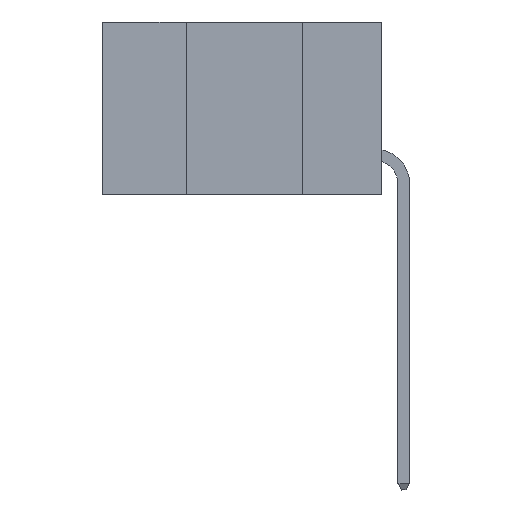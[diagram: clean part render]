
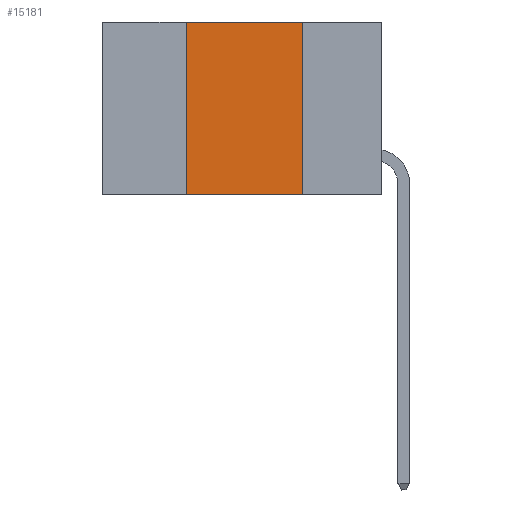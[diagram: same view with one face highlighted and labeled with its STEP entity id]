
A CAD part, left-side view. The second image highlights one B-rep face of the part: STEP entity #15181.
In plain terms, the highlighted planar face has unit normal (-1, 0, 0).
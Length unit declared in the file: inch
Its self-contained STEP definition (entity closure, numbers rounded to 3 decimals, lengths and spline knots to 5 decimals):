
#369 = VECTOR ( 'NONE', #15981, 39.37008 ) ;
#800 = DIRECTION ( 'NONE',  ( 0., 0., -1. ) ) ;
#1093 = DIRECTION ( 'NONE',  ( 0., -1., 0. ) ) ;
#2304 = VECTOR ( 'NONE', #1093, 39.37008 ) ;
#2764 = CARTESIAN_POINT ( 'NONE',  ( 0., 0.42, -0.37 ) ) ;
#4358 = ORIENTED_EDGE ( 'NONE', *, *, #9635, .F. ) ;
#4520 = FACE_OUTER_BOUND ( 'NONE', #13488, .T. ) ;
#5793 = CARTESIAN_POINT ( 'NONE',  ( 0., 0.42, 0. ) ) ;
#6405 = CARTESIAN_POINT ( 'NONE',  ( 0., 0.6, 0. ) ) ;
#6840 = VECTOR ( 'NONE', #7707, 39.37008 ) ;
#6966 = EDGE_CURVE ( 'NONE', #13917, #22539, #12377, .T. ) ;
#7178 = ORIENTED_EDGE ( 'NONE', *, *, #19142, .F. ) ;
#7707 = DIRECTION ( 'NONE',  ( 0., -1., 0. ) ) ;
#7762 = DIRECTION ( 'NONE',  ( 0., 0., 1. ) ) ;
#8821 = VERTEX_POINT ( 'NONE', #2764 ) ;
#9635 = EDGE_CURVE ( 'NONE', #8821, #13917, #11450, .T. ) ;
#9714 = DIRECTION ( 'NONE',  ( 1., 0., 0. ) ) ;
#9797 = PLANE ( 'NONE',  #17584 ) ;
#11450 = LINE ( 'NONE', #18450, #13136 ) ;
#12377 = LINE ( 'NONE', #6405, #2304 ) ;
#13136 = VECTOR ( 'NONE', #7762, 39.37008 ) ;
#13488 = EDGE_LOOP ( 'NONE', ( #7178, #20698, #4358, #21843 ) ) ;
#13760 = CARTESIAN_POINT ( 'NONE',  ( 0., 0.17, -0.37 ) ) ;
#13917 = VERTEX_POINT ( 'NONE', #5793 ) ;
#15181 = ADVANCED_FACE ( 'NONE', ( #4520 ), #9797, .F. ) ;
#15702 = VERTEX_POINT ( 'NONE', #13760 ) ;
#15919 = CARTESIAN_POINT ( 'NONE',  ( 0., 0.17, 0. ) ) ;
#15981 = DIRECTION ( 'NONE',  ( 0., 0., -1. ) ) ;
#16896 = CARTESIAN_POINT ( 'NONE',  ( 0., 0.6, -0.37 ) ) ;
#17584 = AXIS2_PLACEMENT_3D ( 'NONE', #22283, #9714, #800 ) ;
#17777 = CARTESIAN_POINT ( 'NONE',  ( 0., 0.17, 0. ) ) ;
#18450 = CARTESIAN_POINT ( 'NONE',  ( 0., 0.42, 0. ) ) ;
#19142 = EDGE_CURVE ( 'NONE', #22539, #15702, #19927, .T. ) ;
#19927 = LINE ( 'NONE', #15919, #369 ) ;
#20698 = ORIENTED_EDGE ( 'NONE', *, *, #6966, .F. ) ;
#21843 = ORIENTED_EDGE ( 'NONE', *, *, #22896, .T. ) ;
#21914 = LINE ( 'NONE', #16896, #6840 ) ;
#22283 = CARTESIAN_POINT ( 'NONE',  ( 0., 0.6, 0. ) ) ;
#22539 = VERTEX_POINT ( 'NONE', #17777 ) ;
#22896 = EDGE_CURVE ( 'NONE', #8821, #15702, #21914, .T. ) ;
